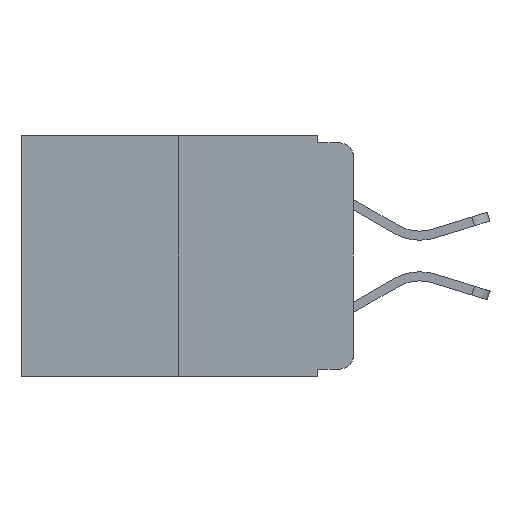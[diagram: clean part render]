
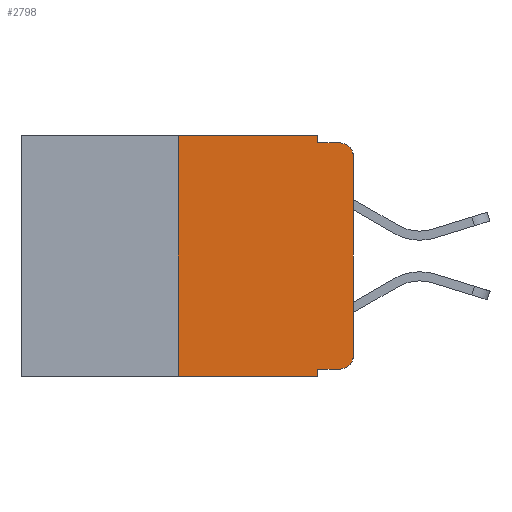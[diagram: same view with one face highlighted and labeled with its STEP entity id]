
A CAD part, left-side view. The second image highlights one B-rep face of the part: STEP entity #2798.
In plain terms, the highlighted planar face has unit normal (-1, 0, 0).
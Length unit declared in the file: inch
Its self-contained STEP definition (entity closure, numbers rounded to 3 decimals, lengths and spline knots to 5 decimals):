
#39 = VERTEX_POINT ( 'NONE', #7086 ) ;
#237 = CARTESIAN_POINT ( 'NONE',  ( 0., 0.051, 0. ) ) ;
#273 = EDGE_CURVE ( 'NONE', #10564, #2573, #2468, .T. ) ;
#439 = EDGE_CURVE ( 'NONE', #39, #10835, #10603, .T. ) ;
#545 = CARTESIAN_POINT ( 'NONE',  ( 0., 0.051, -0.01 ) ) ;
#553 = DIRECTION ( 'NONE',  ( -1., 0., 0. ) ) ;
#591 = DIRECTION ( 'NONE',  ( 0., 0., 1. ) ) ;
#606 = AXIS2_PLACEMENT_3D ( 'NONE', #8194, #1210, #10600 ) ;
#706 = ORIENTED_EDGE ( 'NONE', *, *, #273, .F. ) ;
#1019 = VERTEX_POINT ( 'NONE', #6078 ) ;
#1032 = DIRECTION ( 'NONE',  ( 0., -1., 0. ) ) ;
#1153 = DIRECTION ( 'NONE',  ( 0., 0., -1. ) ) ;
#1210 = DIRECTION ( 'NONE',  ( 1., 0., 0. ) ) ;
#1221 = ORIENTED_EDGE ( 'NONE', *, *, #8439, .F. ) ;
#1428 = CARTESIAN_POINT ( 'NONE',  ( 0., 0.02, -0.03 ) ) ;
#1607 = VECTOR ( 'NONE', #10262, 39.37008 ) ;
#1636 = CARTESIAN_POINT ( 'NONE',  ( 0., 0.051, 0. ) ) ;
#1901 = CARTESIAN_POINT ( 'NONE',  ( 0., 0.02, -0.313 ) ) ;
#1916 = DIRECTION ( 'NONE',  ( 0., 0., 1. ) ) ;
#1958 = CARTESIAN_POINT ( 'NONE',  ( 0., 0.473, 0. ) ) ;
#2468 = LINE ( 'NONE', #237, #5412 ) ;
#2489 = CARTESIAN_POINT ( 'NONE',  ( 0., 0.473, -0.343 ) ) ;
#2573 = VERTEX_POINT ( 'NONE', #6515 ) ;
#2601 = ORIENTED_EDGE ( 'NONE', *, *, #10173, .F. ) ;
#2656 = VERTEX_POINT ( 'NONE', #1636 ) ;
#2686 = VERTEX_POINT ( 'NONE', #3535 ) ;
#2798 = ADVANCED_FACE ( 'NONE', ( #3648 ), #6429, .F. ) ;
#2820 = CIRCLE ( 'NONE', #8810, 0.02 ) ;
#3020 = EDGE_LOOP ( 'NONE', ( #4484, #5478, #11005, #2601, #1221, #11020, #3754, #706, #10980, #6130 ) ) ;
#3153 = DIRECTION ( 'NONE',  ( 0., 0., -1. ) ) ;
#3320 = EDGE_CURVE ( 'NONE', #10564, #3919, #5662, .T. ) ;
#3338 = VERTEX_POINT ( 'NONE', #6208 ) ;
#3356 = LINE ( 'NONE', #545, #5370 ) ;
#3535 = CARTESIAN_POINT ( 'NONE',  ( 0., 0., -0.03 ) ) ;
#3584 = EDGE_CURVE ( 'NONE', #3919, #8535, #2820, .T. ) ;
#3612 = VECTOR ( 'NONE', #1916, 39.37008 ) ;
#3648 = FACE_OUTER_BOUND ( 'NONE', #3020, .T. ) ;
#3652 = CARTESIAN_POINT ( 'NONE',  ( 0., 0., -0.313 ) ) ;
#3754 = ORIENTED_EDGE ( 'NONE', *, *, #8850, .T. ) ;
#3823 = EDGE_CURVE ( 'NONE', #2686, #1019, #5778, .T. ) ;
#3919 = VERTEX_POINT ( 'NONE', #8515 ) ;
#4303 = CARTESIAN_POINT ( 'NONE',  ( 0., 0.051, 0. ) ) ;
#4324 = VECTOR ( 'NONE', #5906, 39.37008 ) ;
#4484 = ORIENTED_EDGE ( 'NONE', *, *, #4794, .T. ) ;
#4794 = EDGE_CURVE ( 'NONE', #8535, #2686, #8178, .T. ) ;
#4885 = VECTOR ( 'NONE', #7963, 39.37008 ) ;
#4983 = LINE ( 'NONE', #4303, #1607 ) ;
#5370 = VECTOR ( 'NONE', #10011, 39.37008 ) ;
#5412 = VECTOR ( 'NONE', #1153, 39.37008 ) ;
#5478 = ORIENTED_EDGE ( 'NONE', *, *, #3823, .T. ) ;
#5662 = LINE ( 'NONE', #8738, #6844 ) ;
#5778 = CIRCLE ( 'NONE', #10489, 0.02 ) ;
#5906 = DIRECTION ( 'NONE',  ( 0., -1., 0. ) ) ;
#6078 = CARTESIAN_POINT ( 'NONE',  ( 0., 0.02, -0.01 ) ) ;
#6130 = ORIENTED_EDGE ( 'NONE', *, *, #3584, .T. ) ;
#6208 = CARTESIAN_POINT ( 'NONE',  ( 0., 0.051, -0.01 ) ) ;
#6429 = PLANE ( 'NONE',  #606 ) ;
#6515 = CARTESIAN_POINT ( 'NONE',  ( 0., 0.051, -0.343 ) ) ;
#6844 = VECTOR ( 'NONE', #1032, 39.37008 ) ;
#7041 = CARTESIAN_POINT ( 'NONE',  ( 0., 0., 0. ) ) ;
#7086 = CARTESIAN_POINT ( 'NONE',  ( 0., 0.25, -0.343 ) ) ;
#7661 = LINE ( 'NONE', #1958, #4885 ) ;
#7906 = DIRECTION ( 'NONE',  ( -1., 0., 0. ) ) ;
#7963 = DIRECTION ( 'NONE',  ( 0., -1., 0. ) ) ;
#8178 = LINE ( 'NONE', #7041, #3612 ) ;
#8194 = CARTESIAN_POINT ( 'NONE',  ( 0., 0.473, 0. ) ) ;
#8287 = CARTESIAN_POINT ( 'NONE',  ( 0., 0.25, 0. ) ) ;
#8439 = EDGE_CURVE ( 'NONE', #10835, #2656, #7661, .T. ) ;
#8515 = CARTESIAN_POINT ( 'NONE',  ( 0., 0.02, -0.333 ) ) ;
#8535 = VERTEX_POINT ( 'NONE', #3652 ) ;
#8738 = CARTESIAN_POINT ( 'NONE',  ( 0., 0.051, -0.333 ) ) ;
#8810 = AXIS2_PLACEMENT_3D ( 'NONE', #1901, #7906, #9827 ) ;
#8850 = EDGE_CURVE ( 'NONE', #39, #2573, #8872, .T. ) ;
#8872 = LINE ( 'NONE', #2489, #4324 ) ;
#9116 = CARTESIAN_POINT ( 'NONE',  ( 0., 0.051, -0.333 ) ) ;
#9438 = CARTESIAN_POINT ( 'NONE',  ( 0., 0.25, 0. ) ) ;
#9827 = DIRECTION ( 'NONE',  ( 0., 0., -1. ) ) ;
#9970 = EDGE_CURVE ( 'NONE', #3338, #1019, #3356, .T. ) ;
#10011 = DIRECTION ( 'NONE',  ( 0., -1., 0. ) ) ;
#10173 = EDGE_CURVE ( 'NONE', #2656, #3338, #4983, .T. ) ;
#10262 = DIRECTION ( 'NONE',  ( 0., 0., -1. ) ) ;
#10461 = VECTOR ( 'NONE', #591, 39.37008 ) ;
#10489 = AXIS2_PLACEMENT_3D ( 'NONE', #1428, #553, #3153 ) ;
#10564 = VERTEX_POINT ( 'NONE', #9116 ) ;
#10600 = DIRECTION ( 'NONE',  ( 0., 0., -1. ) ) ;
#10603 = LINE ( 'NONE', #8287, #10461 ) ;
#10835 = VERTEX_POINT ( 'NONE', #9438 ) ;
#10980 = ORIENTED_EDGE ( 'NONE', *, *, #3320, .T. ) ;
#11005 = ORIENTED_EDGE ( 'NONE', *, *, #9970, .F. ) ;
#11020 = ORIENTED_EDGE ( 'NONE', *, *, #439, .F. ) ;
